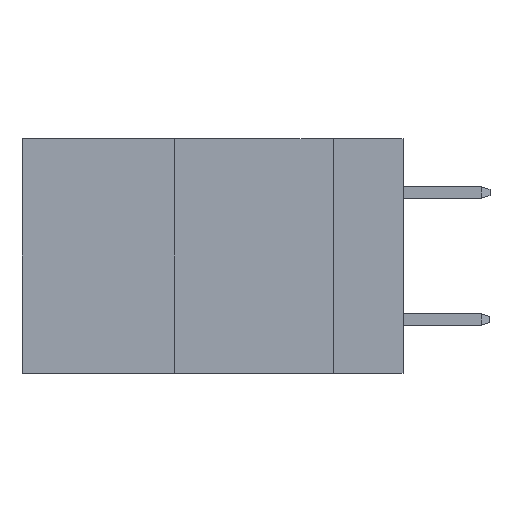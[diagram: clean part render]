
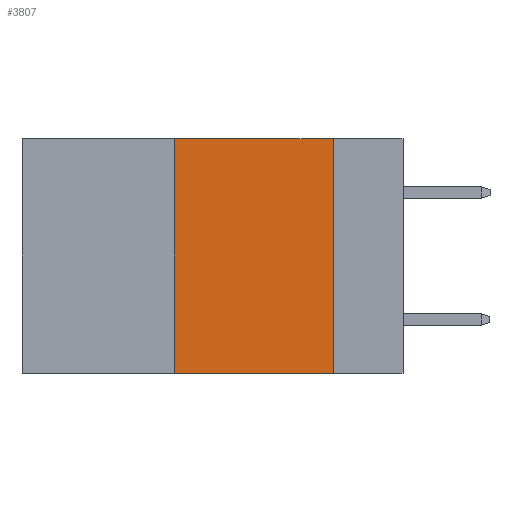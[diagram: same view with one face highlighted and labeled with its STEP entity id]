
A CAD part, left-side view. The second image highlights one B-rep face of the part: STEP entity #3807.
In plain terms, the highlighted planar face has unit normal (-1, 0, 0).
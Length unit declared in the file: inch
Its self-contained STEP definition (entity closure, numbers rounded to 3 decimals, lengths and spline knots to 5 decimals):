
#128 = EDGE_CURVE ( 'NONE', #11586, #9176, #7883, .T. ) ;
#202 = LINE ( 'NONE', #260, #7917 ) ;
#260 = CARTESIAN_POINT ( 'NONE',  ( 0., 0.6, 0. ) ) ;
#454 = VECTOR ( 'NONE', #4460, 39.37008 ) ;
#698 = ORIENTED_EDGE ( 'NONE', *, *, #8576, .F. ) ;
#721 = CARTESIAN_POINT ( 'NONE',  ( 0., 0.11, 0. ) ) ;
#1162 = DIRECTION ( 'NONE',  ( 1., 0., 0. ) ) ;
#1539 = DIRECTION ( 'NONE',  ( 0., -1., 0. ) ) ;
#1777 = DIRECTION ( 'NONE',  ( 0., 0., -1. ) ) ;
#1785 = VECTOR ( 'NONE', #1539, 39.37008 ) ;
#2066 = ORIENTED_EDGE ( 'NONE', *, *, #6275, .F. ) ;
#2467 = CARTESIAN_POINT ( 'NONE',  ( 0., 0.36, -0.37 ) ) ;
#2509 = EDGE_LOOP ( 'NONE', ( #7110, #2066, #698, #8337 ) ) ;
#2734 = DIRECTION ( 'NONE',  ( 0., -1., 0. ) ) ;
#3798 = VECTOR ( 'NONE', #1777, 39.37008 ) ;
#3807 = ADVANCED_FACE ( 'NONE', ( #5609 ), #6445, .F. ) ;
#3935 = DIRECTION ( 'NONE',  ( 0., 0., -1. ) ) ;
#4460 = DIRECTION ( 'NONE',  ( 0., 0., 1. ) ) ;
#5609 = FACE_OUTER_BOUND ( 'NONE', #2509, .T. ) ;
#6205 = AXIS2_PLACEMENT_3D ( 'NONE', #8269, #1162, #3935 ) ;
#6239 = CARTESIAN_POINT ( 'NONE',  ( 0., 0.11, 0. ) ) ;
#6275 = EDGE_CURVE ( 'NONE', #7005, #7957, #202, .T. ) ;
#6445 = PLANE ( 'NONE',  #6205 ) ;
#7005 = VERTEX_POINT ( 'NONE', #7625 ) ;
#7008 = CARTESIAN_POINT ( 'NONE',  ( 0., 0.6, -0.37 ) ) ;
#7057 = EDGE_CURVE ( 'NONE', #7957, #9176, #10558, .T. ) ;
#7110 = ORIENTED_EDGE ( 'NONE', *, *, #7057, .F. ) ;
#7625 = CARTESIAN_POINT ( 'NONE',  ( 0., 0.36, 0. ) ) ;
#7883 = LINE ( 'NONE', #7008, #1785 ) ;
#7917 = VECTOR ( 'NONE', #2734, 39.37008 ) ;
#7957 = VERTEX_POINT ( 'NONE', #721 ) ;
#8269 = CARTESIAN_POINT ( 'NONE',  ( 0., 0.6, 0. ) ) ;
#8337 = ORIENTED_EDGE ( 'NONE', *, *, #128, .T. ) ;
#8576 = EDGE_CURVE ( 'NONE', #11586, #7005, #10988, .T. ) ;
#8992 = CARTESIAN_POINT ( 'NONE',  ( 0., 0.36, 0. ) ) ;
#9076 = CARTESIAN_POINT ( 'NONE',  ( 0., 0.11, -0.37 ) ) ;
#9176 = VERTEX_POINT ( 'NONE', #9076 ) ;
#10558 = LINE ( 'NONE', #6239, #3798 ) ;
#10988 = LINE ( 'NONE', #8992, #454 ) ;
#11586 = VERTEX_POINT ( 'NONE', #2467 ) ;
